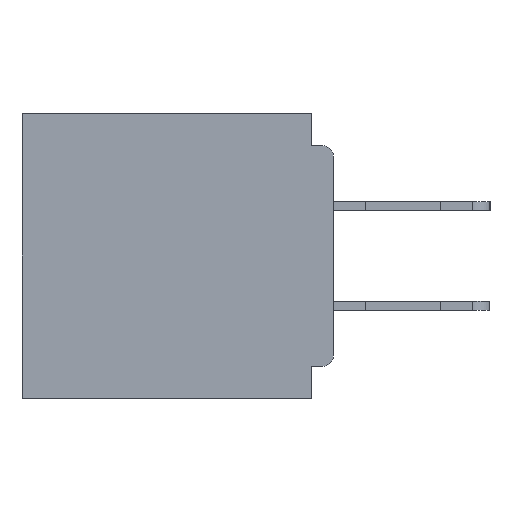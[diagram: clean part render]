
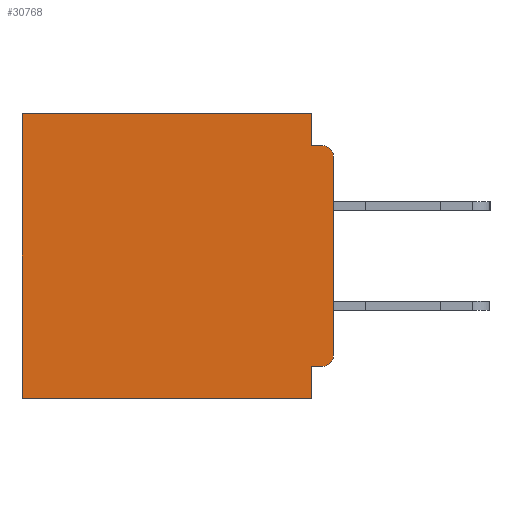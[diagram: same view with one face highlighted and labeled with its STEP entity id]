
A CAD part, left-side view. The second image highlights one B-rep face of the part: STEP entity #30768.
In plain terms, the highlighted planar face has unit normal (-1, 0, 0).
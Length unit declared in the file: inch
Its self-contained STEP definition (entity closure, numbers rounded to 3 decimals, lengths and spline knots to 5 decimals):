
#84 = LINE ( 'NONE', #7850, #11255 ) ;
#1983 = ORIENTED_EDGE ( 'NONE', *, *, #25447, .F. ) ;
#2403 = VERTEX_POINT ( 'NONE', #3676 ) ;
#2711 = DIRECTION ( 'NONE',  ( 0., 0., -1. ) ) ;
#2859 = VECTOR ( 'NONE', #48167, 39.37008 ) ;
#3676 = CARTESIAN_POINT ( 'NONE',  ( 0.3, 0.031, -0.4 ) ) ;
#4083 = EDGE_CURVE ( 'NONE', #35500, #2403, #19855, .T. ) ;
#4179 = LINE ( 'NONE', #52136, #2859 ) ;
#4922 = CARTESIAN_POINT ( 'NONE',  ( 0.3, 0.031, -0.355 ) ) ;
#5319 = CARTESIAN_POINT ( 'NONE',  ( 0.3, 0.015, -0.355 ) ) ;
#6681 = VECTOR ( 'NONE', #44095, 39.37008 ) ;
#6818 = EDGE_LOOP ( 'NONE', ( #20611, #44160, #1983, #31945, #39851, #53178, #34700, #29533, #49049, #19131 ) ) ;
#7092 = VECTOR ( 'NONE', #43442, 39.37008 ) ;
#7247 = DIRECTION ( 'NONE',  ( -1., 0., 0. ) ) ;
#7551 = LINE ( 'NONE', #26943, #27146 ) ;
#7850 = CARTESIAN_POINT ( 'NONE',  ( 0.3, 0., -0.4 ) ) ;
#8175 = VERTEX_POINT ( 'NONE', #11662 ) ;
#8748 = DIRECTION ( 'NONE',  ( 1., 0., 0. ) ) ;
#9566 = FACE_OUTER_BOUND ( 'NONE', #6818, .T. ) ;
#11255 = VECTOR ( 'NONE', #36954, 39.37008 ) ;
#11662 = CARTESIAN_POINT ( 'NONE',  ( 0.3, 0.031, -0.045 ) ) ;
#11744 = DIRECTION ( 'NONE',  ( 0., 0., -1. ) ) ;
#11839 = EDGE_CURVE ( 'NONE', #50463, #29085, #34688, .T. ) ;
#12557 = VECTOR ( 'NONE', #2711, 39.37008 ) ;
#13625 = CARTESIAN_POINT ( 'NONE',  ( 0.3, 0.437, -0.4 ) ) ;
#14581 = DIRECTION ( 'NONE',  ( 0., 1., 0. ) ) ;
#15186 = CARTESIAN_POINT ( 'NONE',  ( 0.3, 0., -0.4 ) ) ;
#16235 = LINE ( 'NONE', #13625, #46570 ) ;
#17275 = EDGE_CURVE ( 'NONE', #43493, #34440, #16235, .T. ) ;
#17395 = CARTESIAN_POINT ( 'NONE',  ( 0.3, 0.031, 0. ) ) ;
#17741 = EDGE_CURVE ( 'NONE', #22480, #29085, #38200, .T. ) ;
#18286 = LINE ( 'NONE', #26883, #7092 ) ;
#18535 = VERTEX_POINT ( 'NONE', #17395 ) ;
#18803 = AXIS2_PLACEMENT_3D ( 'NONE', #45880, #8748, #37806 ) ;
#19131 = ORIENTED_EDGE ( 'NONE', *, *, #17741, .T. ) ;
#19855 = LINE ( 'NONE', #33551, #51421 ) ;
#20611 = ORIENTED_EDGE ( 'NONE', *, *, #11839, .F. ) ;
#20639 = CARTESIAN_POINT ( 'NONE',  ( 0.3, 0.015, -0.045 ) ) ;
#22258 = CARTESIAN_POINT ( 'NONE',  ( 0.3, 0.437, -0.4 ) ) ;
#22347 = CARTESIAN_POINT ( 'NONE',  ( 0.3, 0., -0.06 ) ) ;
#22480 = VERTEX_POINT ( 'NONE', #5319 ) ;
#23658 = LINE ( 'NONE', #27767, #12557 ) ;
#24894 = CARTESIAN_POINT ( 'NONE',  ( 0.3, 0.015, -0.34 ) ) ;
#25344 = CARTESIAN_POINT ( 'NONE',  ( 0.3, 0.437, 0. ) ) ;
#25447 = EDGE_CURVE ( 'NONE', #8175, #29358, #18286, .T. ) ;
#26883 = CARTESIAN_POINT ( 'NONE',  ( 0.3, 0., -0.045 ) ) ;
#26943 = CARTESIAN_POINT ( 'NONE',  ( 0.3, 0., 0. ) ) ;
#27131 = CARTESIAN_POINT ( 'NONE',  ( 0.3, 0., -0.34 ) ) ;
#27146 = VECTOR ( 'NONE', #14581, 39.37008 ) ;
#27650 = EDGE_CURVE ( 'NONE', #2403, #34440, #84, .T. ) ;
#27767 = CARTESIAN_POINT ( 'NONE',  ( 0.3, 0.031, 0. ) ) ;
#29080 = DIRECTION ( 'NONE',  ( 0., 0., -1. ) ) ;
#29085 = VERTEX_POINT ( 'NONE', #27131 ) ;
#29358 = VERTEX_POINT ( 'NONE', #20639 ) ;
#29533 = ORIENTED_EDGE ( 'NONE', *, *, #4083, .F. ) ;
#30768 = ADVANCED_FACE ( 'NONE', ( #9566 ), #33668, .F. ) ;
#30994 = EDGE_CURVE ( 'NONE', #18535, #43493, #7551, .T. ) ;
#31945 = ORIENTED_EDGE ( 'NONE', *, *, #39637, .F. ) ;
#32228 = CARTESIAN_POINT ( 'NONE',  ( 0.3, 0.015, -0.06 ) ) ;
#33551 = CARTESIAN_POINT ( 'NONE',  ( 0.3, 0.031, -0.4 ) ) ;
#33668 = PLANE ( 'NONE',  #18803 ) ;
#34440 = VERTEX_POINT ( 'NONE', #22258 ) ;
#34688 = LINE ( 'NONE', #15186, #6681 ) ;
#34700 = ORIENTED_EDGE ( 'NONE', *, *, #27650, .F. ) ;
#35500 = VERTEX_POINT ( 'NONE', #4922 ) ;
#36351 = DIRECTION ( 'NONE',  ( 0., 0., -1. ) ) ;
#36954 = DIRECTION ( 'NONE',  ( 0., 1., 0. ) ) ;
#37806 = DIRECTION ( 'NONE',  ( 0., 0., -1. ) ) ;
#38200 = CIRCLE ( 'NONE', #51009, 0.015 ) ;
#38470 = DIRECTION ( 'NONE',  ( 0., 0., -1. ) ) ;
#39637 = EDGE_CURVE ( 'NONE', #18535, #8175, #23658, .T. ) ;
#39851 = ORIENTED_EDGE ( 'NONE', *, *, #30994, .T. ) ;
#43148 = CIRCLE ( 'NONE', #47364, 0.015 ) ;
#43442 = DIRECTION ( 'NONE',  ( 0., -1., 0. ) ) ;
#43493 = VERTEX_POINT ( 'NONE', #25344 ) ;
#44095 = DIRECTION ( 'NONE',  ( 0., 0., -1. ) ) ;
#44160 = ORIENTED_EDGE ( 'NONE', *, *, #48133, .T. ) ;
#45880 = CARTESIAN_POINT ( 'NONE',  ( 0.3, 0., -0.4 ) ) ;
#46570 = VECTOR ( 'NONE', #38470, 39.37008 ) ;
#47364 = AXIS2_PLACEMENT_3D ( 'NONE', #32228, #7247, #36351 ) ;
#48133 = EDGE_CURVE ( 'NONE', #50463, #29358, #43148, .T. ) ;
#48167 = DIRECTION ( 'NONE',  ( 0., 1., 0. ) ) ;
#49049 = ORIENTED_EDGE ( 'NONE', *, *, #52648, .F. ) ;
#50463 = VERTEX_POINT ( 'NONE', #22347 ) ;
#51009 = AXIS2_PLACEMENT_3D ( 'NONE', #24894, #53699, #29080 ) ;
#51421 = VECTOR ( 'NONE', #11744, 39.37008 ) ;
#52136 = CARTESIAN_POINT ( 'NONE',  ( 0.3, 0., -0.355 ) ) ;
#52648 = EDGE_CURVE ( 'NONE', #22480, #35500, #4179, .T. ) ;
#53178 = ORIENTED_EDGE ( 'NONE', *, *, #17275, .T. ) ;
#53699 = DIRECTION ( 'NONE',  ( -1., 0., 0. ) ) ;
